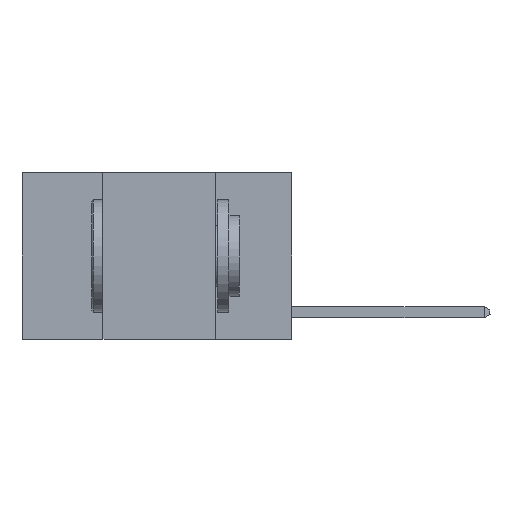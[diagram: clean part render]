
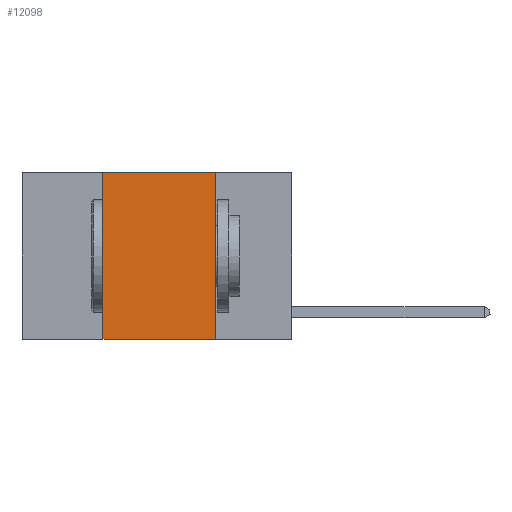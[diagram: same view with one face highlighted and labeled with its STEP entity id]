
A CAD part, left-side view. The second image highlights one B-rep face of the part: STEP entity #12098.
In plain terms, the highlighted planar face has unit normal (-1, 0, 0).
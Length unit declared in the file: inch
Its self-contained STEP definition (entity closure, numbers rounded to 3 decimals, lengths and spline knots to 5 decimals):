
#256 = CARTESIAN_POINT ( 'NONE',  ( 0., 0.6, 0. ) ) ;
#573 = VERTEX_POINT ( 'NONE', #3323 ) ;
#1674 = VECTOR ( 'NONE', #5018, 39.37008 ) ;
#2470 = EDGE_CURVE ( 'NONE', #573, #22450, #21265, .T. ) ;
#2966 = DIRECTION ( 'NONE',  ( 0., 0., 1. ) ) ;
#3323 = CARTESIAN_POINT ( 'NONE',  ( 0., 0.42, -0.37 ) ) ;
#4457 = EDGE_CURVE ( 'NONE', #22450, #4996, #21435, .T. ) ;
#4766 = DIRECTION ( 'NONE',  ( 0., -1., 0. ) ) ;
#4996 = VERTEX_POINT ( 'NONE', #8014 ) ;
#5018 = DIRECTION ( 'NONE',  ( 0., 0., -1. ) ) ;
#5493 = PLANE ( 'NONE',  #13811 ) ;
#6284 = DIRECTION ( 'NONE',  ( 0., -1., 0. ) ) ;
#6509 = VERTEX_POINT ( 'NONE', #8581 ) ;
#6770 = CARTESIAN_POINT ( 'NONE',  ( 0., 0.17, 0. ) ) ;
#7257 = DIRECTION ( 'NONE',  ( 0., 0., -1. ) ) ;
#7407 = VECTOR ( 'NONE', #6284, 39.37008 ) ;
#7422 = VECTOR ( 'NONE', #2966, 39.37008 ) ;
#8014 = CARTESIAN_POINT ( 'NONE',  ( 0., 0.17, 0. ) ) ;
#8156 = EDGE_CURVE ( 'NONE', #573, #6509, #19074, .T. ) ;
#8581 = CARTESIAN_POINT ( 'NONE',  ( 0., 0.17, -0.37 ) ) ;
#10007 = CARTESIAN_POINT ( 'NONE',  ( 0., 0.42, 0. ) ) ;
#11890 = ORIENTED_EDGE ( 'NONE', *, *, #2470, .F. ) ;
#12098 = ADVANCED_FACE ( 'NONE', ( #15923 ), #5493, .F. ) ;
#13811 = AXIS2_PLACEMENT_3D ( 'NONE', #256, #17679, #7257 ) ;
#14043 = ORIENTED_EDGE ( 'NONE', *, *, #8156, .T. ) ;
#15071 = CARTESIAN_POINT ( 'NONE',  ( 0., 0.42, 0. ) ) ;
#15923 = FACE_OUTER_BOUND ( 'NONE', #19668, .T. ) ;
#16914 = CARTESIAN_POINT ( 'NONE',  ( 0., 0.6, 0. ) ) ;
#17679 = DIRECTION ( 'NONE',  ( 1., 0., 0. ) ) ;
#18464 = CARTESIAN_POINT ( 'NONE',  ( 0., 0.6, -0.37 ) ) ;
#19074 = LINE ( 'NONE', #18464, #7407 ) ;
#19398 = EDGE_CURVE ( 'NONE', #4996, #6509, #20122, .T. ) ;
#19668 = EDGE_LOOP ( 'NONE', ( #20794, #21065, #11890, #14043 ) ) ;
#20122 = LINE ( 'NONE', #6770, #1674 ) ;
#20794 = ORIENTED_EDGE ( 'NONE', *, *, #19398, .F. ) ;
#21065 = ORIENTED_EDGE ( 'NONE', *, *, #4457, .F. ) ;
#21265 = LINE ( 'NONE', #15071, #7422 ) ;
#21435 = LINE ( 'NONE', #16914, #21991 ) ;
#21991 = VECTOR ( 'NONE', #4766, 39.37008 ) ;
#22450 = VERTEX_POINT ( 'NONE', #10007 ) ;
